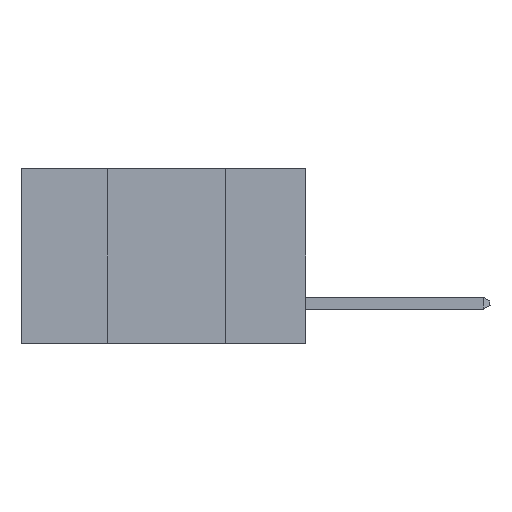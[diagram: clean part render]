
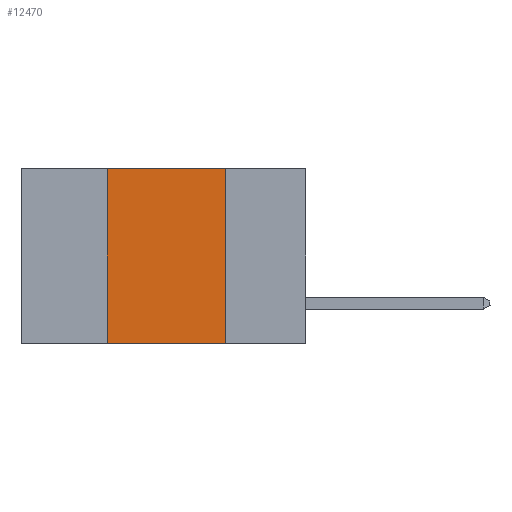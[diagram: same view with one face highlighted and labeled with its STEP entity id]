
A CAD part, left-side view. The second image highlights one B-rep face of the part: STEP entity #12470.
In plain terms, the highlighted planar face has unit normal (-1, 0, 0).
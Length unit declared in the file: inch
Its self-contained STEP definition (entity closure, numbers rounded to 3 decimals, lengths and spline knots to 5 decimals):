
#78 = VECTOR ( 'NONE', #12581, 39.37008 ) ;
#139 = CARTESIAN_POINT ( 'NONE',  ( 0., 0.42, -0.37 ) ) ;
#279 = VERTEX_POINT ( 'NONE', #8816 ) ;
#473 = PLANE ( 'NONE',  #4645 ) ;
#676 = CARTESIAN_POINT ( 'NONE',  ( 0., 0.17, -0.37 ) ) ;
#1175 = LINE ( 'NONE', #4687, #78 ) ;
#1266 = ORIENTED_EDGE ( 'NONE', *, *, #9361, .F. ) ;
#1380 = EDGE_CURVE ( 'NONE', #9023, #279, #10771, .T. ) ;
#1516 = EDGE_CURVE ( 'NONE', #12250, #9023, #6254, .T. ) ;
#1551 = CARTESIAN_POINT ( 'NONE',  ( 0., 0.42, 0. ) ) ;
#1812 = EDGE_LOOP ( 'NONE', ( #1266, #6983, #8949, #10174 ) ) ;
#2251 = VECTOR ( 'NONE', #6160, 39.37008 ) ;
#2532 = VERTEX_POINT ( 'NONE', #676 ) ;
#2578 = EDGE_CURVE ( 'NONE', #12250, #2532, #1175, .T. ) ;
#3516 = LINE ( 'NONE', #6072, #2251 ) ;
#3587 = VECTOR ( 'NONE', #11540, 39.37008 ) ;
#4645 = AXIS2_PLACEMENT_3D ( 'NONE', #6369, #9504, #8467 ) ;
#4687 = CARTESIAN_POINT ( 'NONE',  ( 0., 0.6, -0.37 ) ) ;
#6072 = CARTESIAN_POINT ( 'NONE',  ( 0., 0.17, 0. ) ) ;
#6160 = DIRECTION ( 'NONE',  ( 0., 0., -1. ) ) ;
#6254 = LINE ( 'NONE', #1551, #3587 ) ;
#6287 = CARTESIAN_POINT ( 'NONE',  ( 0., 0.6, 0. ) ) ;
#6369 = CARTESIAN_POINT ( 'NONE',  ( 0., 0.6, 0. ) ) ;
#6718 = FACE_OUTER_BOUND ( 'NONE', #1812, .T. ) ;
#6983 = ORIENTED_EDGE ( 'NONE', *, *, #1380, .F. ) ;
#8467 = DIRECTION ( 'NONE',  ( 0., 0., -1. ) ) ;
#8816 = CARTESIAN_POINT ( 'NONE',  ( 0., 0.17, 0. ) ) ;
#8949 = ORIENTED_EDGE ( 'NONE', *, *, #1516, .F. ) ;
#9023 = VERTEX_POINT ( 'NONE', #12393 ) ;
#9361 = EDGE_CURVE ( 'NONE', #279, #2532, #3516, .T. ) ;
#9504 = DIRECTION ( 'NONE',  ( 1., 0., 0. ) ) ;
#10174 = ORIENTED_EDGE ( 'NONE', *, *, #2578, .T. ) ;
#10336 = DIRECTION ( 'NONE',  ( 0., -1., 0. ) ) ;
#10771 = LINE ( 'NONE', #6287, #12491 ) ;
#11540 = DIRECTION ( 'NONE',  ( 0., 0., 1. ) ) ;
#12250 = VERTEX_POINT ( 'NONE', #139 ) ;
#12393 = CARTESIAN_POINT ( 'NONE',  ( 0., 0.42, 0. ) ) ;
#12470 = ADVANCED_FACE ( 'NONE', ( #6718 ), #473, .F. ) ;
#12491 = VECTOR ( 'NONE', #10336, 39.37008 ) ;
#12581 = DIRECTION ( 'NONE',  ( 0., -1., 0. ) ) ;
